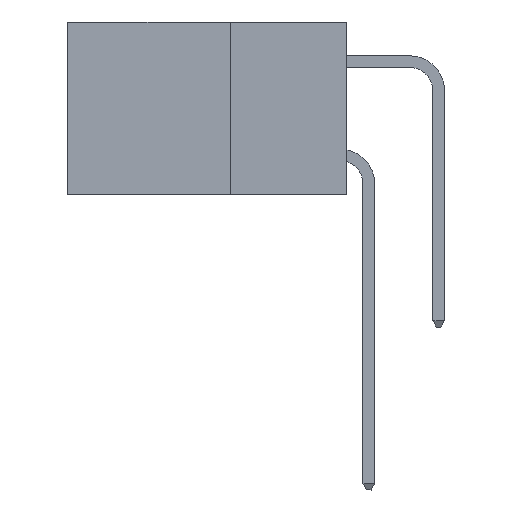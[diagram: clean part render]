
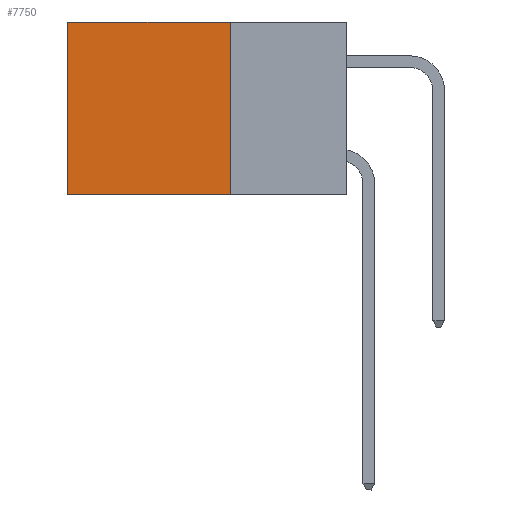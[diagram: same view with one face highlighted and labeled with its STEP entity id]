
A CAD part, left-side view. The second image highlights one B-rep face of the part: STEP entity #7750.
In plain terms, the highlighted planar face has unit normal (-1, 0, 0).
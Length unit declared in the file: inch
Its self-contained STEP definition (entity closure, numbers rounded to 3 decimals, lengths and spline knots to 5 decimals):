
#539 = ORIENTED_EDGE ( 'NONE', *, *, #9924, .F. ) ;
#999 = LINE ( 'NONE', #9071, #4036 ) ;
#1809 = CARTESIAN_POINT ( 'NONE',  ( 0.2875, 0.25, 0. ) ) ;
#1964 = VERTEX_POINT ( 'NONE', #7315 ) ;
#2591 = LINE ( 'NONE', #7040, #7893 ) ;
#4036 = VECTOR ( 'NONE', #6178, 39.37008 ) ;
#4403 = DIRECTION ( 'NONE',  ( 0., 0., -1. ) ) ;
#5818 = LINE ( 'NONE', #1809, #6846 ) ;
#6111 = CARTESIAN_POINT ( 'NONE',  ( 0.2875, 0.25, 0. ) ) ;
#6178 = DIRECTION ( 'NONE',  ( 0., 0., -1. ) ) ;
#6605 = ORIENTED_EDGE ( 'NONE', *, *, #8304, .T. ) ;
#6846 = VECTOR ( 'NONE', #4403, 39.37008 ) ;
#7040 = CARTESIAN_POINT ( 'NONE',  ( 0.2875, 0.25, -0.37 ) ) ;
#7229 = ORIENTED_EDGE ( 'NONE', *, *, #11372, .F. ) ;
#7315 = CARTESIAN_POINT ( 'NONE',  ( 0.2875, 0.25, 0. ) ) ;
#7750 = ADVANCED_FACE ( 'NONE', ( #11158 ), #14143, .F. ) ;
#7893 = VECTOR ( 'NONE', #11022, 39.37008 ) ;
#8304 = EDGE_CURVE ( 'NONE', #8556, #16419, #999, .T. ) ;
#8556 = VERTEX_POINT ( 'NONE', #17353 ) ;
#8687 = DIRECTION ( 'NONE',  ( 1., 0., 0. ) ) ;
#8868 = ORIENTED_EDGE ( 'NONE', *, *, #16167, .T. ) ;
#9071 = CARTESIAN_POINT ( 'NONE',  ( 0.2875, 0.6, 0. ) ) ;
#9687 = VERTEX_POINT ( 'NONE', #15875 ) ;
#9924 = EDGE_CURVE ( 'NONE', #1964, #9687, #5818, .T. ) ;
#11022 = DIRECTION ( 'NONE',  ( 0., 1., 0. ) ) ;
#11028 = VECTOR ( 'NONE', #15025, 39.37008 ) ;
#11158 = FACE_OUTER_BOUND ( 'NONE', #12574, .T. ) ;
#11372 = EDGE_CURVE ( 'NONE', #9687, #16419, #2591, .T. ) ;
#11505 = DIRECTION ( 'NONE',  ( 0., 0., -1. ) ) ;
#12080 = CARTESIAN_POINT ( 'NONE',  ( 0.2875, 0.6, -0.37 ) ) ;
#12563 = LINE ( 'NONE', #12650, #11028 ) ;
#12574 = EDGE_LOOP ( 'NONE', ( #6605, #7229, #539, #8868 ) ) ;
#12650 = CARTESIAN_POINT ( 'NONE',  ( 0.2875, 0.25, 0. ) ) ;
#14143 = PLANE ( 'NONE',  #16853 ) ;
#15025 = DIRECTION ( 'NONE',  ( 0., 1., 0. ) ) ;
#15875 = CARTESIAN_POINT ( 'NONE',  ( 0.2875, 0.25, -0.37 ) ) ;
#16167 = EDGE_CURVE ( 'NONE', #1964, #8556, #12563, .T. ) ;
#16419 = VERTEX_POINT ( 'NONE', #12080 ) ;
#16853 = AXIS2_PLACEMENT_3D ( 'NONE', #6111, #8687, #11505 ) ;
#17353 = CARTESIAN_POINT ( 'NONE',  ( 0.2875, 0.6, 0. ) ) ;
